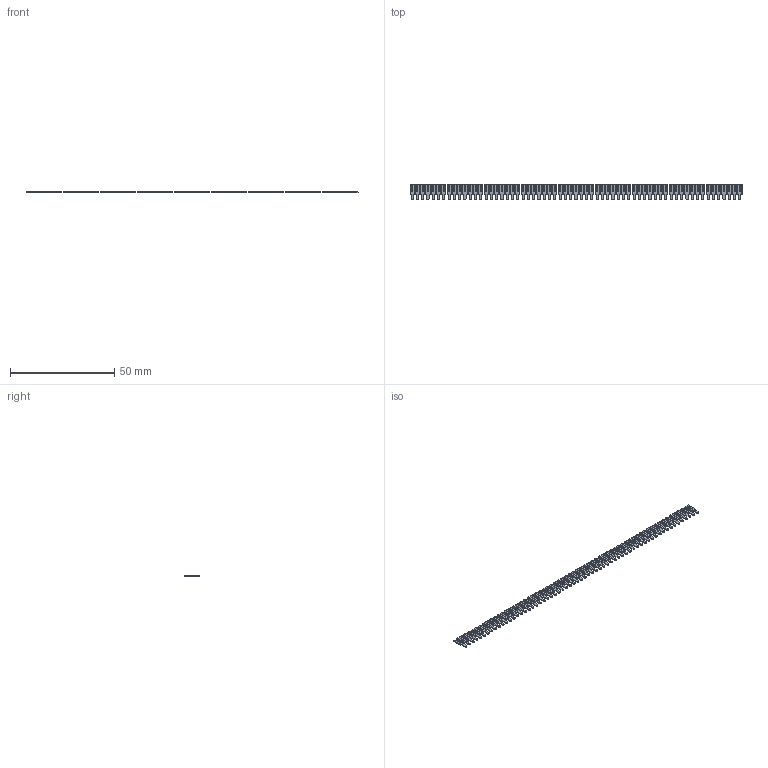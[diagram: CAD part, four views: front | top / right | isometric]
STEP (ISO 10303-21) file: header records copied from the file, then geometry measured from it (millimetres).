
FILE_DESCRIPTION (( 'STEP AP203' ), '1' );
FILE_NAME ('103-063-253-100.STEP', '2020-04-16T16:38:34', ( '' ), ( '' ), 'SwSTEP 2.0', 'SolidWorks 2016', '' );
FILE_SCHEMA (( 'CONFIG_CONTROL_DESIGN' ));
Length unit declared in the file: inch
Products named in the file (2): 100-290-001_100-290-253; 103-063-253-100
Assembly tree (63 placements, depth 2):
  103-063-253-100
    100-290-001_100-290-253  x63
Bounding box: 159.51 x 7.62 x 0.51 mm (x, y, z)
Volume: 347.6 mm3; surface area: 2167.6 mm2
Topology: 63 solids, 63 shells, 1260 faces, 3402 edges, 2268 vertices
Faces by surface type: plane 1197, cylinder 63
Entity records: 2804 total; most frequent: DIRECTION 228, CARTESIAN_POINT 176, DATE_AND_TIME 136, CALENDAR_DATE 136, COORDINATED_UNIVERSAL_TIME_OFFSET 136, LOCAL_TIME 136, ORIENTED_EDGE 108, AXIS2_PLACEMENT_3D 88
